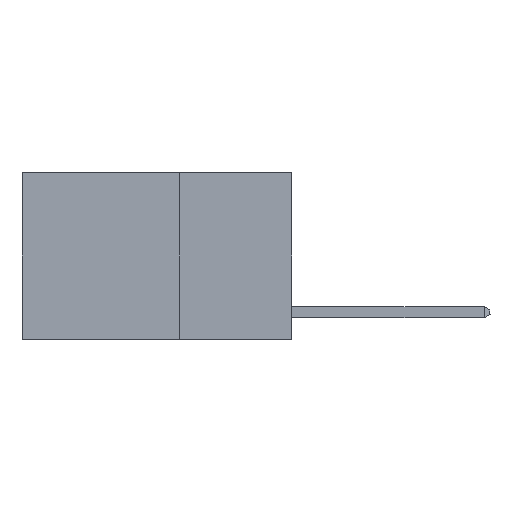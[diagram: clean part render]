
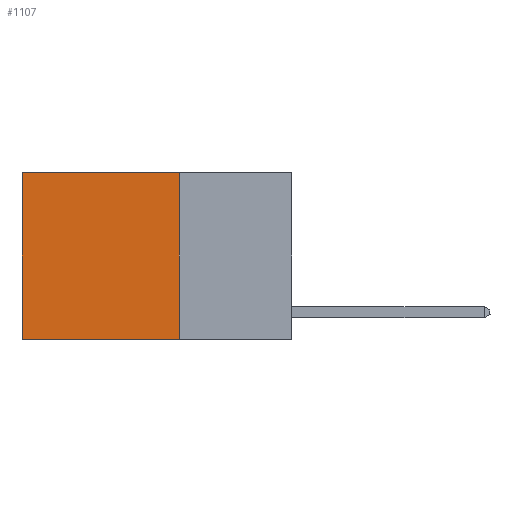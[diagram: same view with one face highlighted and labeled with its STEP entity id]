
A CAD part, left-side view. The second image highlights one B-rep face of the part: STEP entity #1107.
In plain terms, the highlighted planar face has unit normal (-1, 0, 0).
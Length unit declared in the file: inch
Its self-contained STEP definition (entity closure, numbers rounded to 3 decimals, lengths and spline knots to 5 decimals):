
#241 = LINE ( 'NONE', #2129, #24975 ) ;
#943 = FACE_OUTER_BOUND ( 'NONE', #8491, .T. ) ;
#1107 = ADVANCED_FACE ( 'NONE', ( #943 ), #19808, .F. ) ;
#1200 = EDGE_CURVE ( 'NONE', #25346, #14595, #7645, .T. ) ;
#2129 = CARTESIAN_POINT ( 'NONE',  ( 0.2625, 0.25, 0. ) ) ;
#2719 = CARTESIAN_POINT ( 'NONE',  ( 0.2625, 0.25, 0. ) ) ;
#2790 = AXIS2_PLACEMENT_3D ( 'NONE', #7465, #24281, #11390 ) ;
#3312 = ORIENTED_EDGE ( 'NONE', *, *, #1200, .T. ) ;
#3398 = CARTESIAN_POINT ( 'NONE',  ( 0.2625, 0.25, 0. ) ) ;
#6234 = CARTESIAN_POINT ( 'NONE',  ( 0.2625, 0.6, 0. ) ) ;
#7453 = VERTEX_POINT ( 'NONE', #2719 ) ;
#7465 = CARTESIAN_POINT ( 'NONE',  ( 0.2625, 0.25, 0. ) ) ;
#7645 = LINE ( 'NONE', #26067, #15095 ) ;
#7686 = VECTOR ( 'NONE', #24689, 39.37008 ) ;
#8491 = EDGE_LOOP ( 'NONE', ( #3312, #26385, #12675, #25657 ) ) ;
#10450 = DIRECTION ( 'NONE',  ( 0., 0., -1. ) ) ;
#11027 = EDGE_CURVE ( 'NONE', #7453, #25346, #13471, .T. ) ;
#11390 = DIRECTION ( 'NONE',  ( 0., 0., -1. ) ) ;
#12449 = CARTESIAN_POINT ( 'NONE',  ( 0.2625, 0.25, -0.37 ) ) ;
#12675 = ORIENTED_EDGE ( 'NONE', *, *, #24323, .F. ) ;
#13471 = LINE ( 'NONE', #3398, #19526 ) ;
#13715 = DIRECTION ( 'NONE',  ( 0., 0., -1. ) ) ;
#14595 = VERTEX_POINT ( 'NONE', #20973 ) ;
#15095 = VECTOR ( 'NONE', #13715, 39.37008 ) ;
#15436 = VERTEX_POINT ( 'NONE', #12449 ) ;
#16542 = LINE ( 'NONE', #18158, #7686 ) ;
#18158 = CARTESIAN_POINT ( 'NONE',  ( 0.2625, 0.25, -0.37 ) ) ;
#19526 = VECTOR ( 'NONE', #24349, 39.37008 ) ;
#19808 = PLANE ( 'NONE',  #2790 ) ;
#20973 = CARTESIAN_POINT ( 'NONE',  ( 0.2625, 0.6, -0.37 ) ) ;
#24281 = DIRECTION ( 'NONE',  ( 1., 0., 0. ) ) ;
#24323 = EDGE_CURVE ( 'NONE', #7453, #15436, #241, .T. ) ;
#24349 = DIRECTION ( 'NONE',  ( 0., 1., 0. ) ) ;
#24689 = DIRECTION ( 'NONE',  ( 0., 1., 0. ) ) ;
#24975 = VECTOR ( 'NONE', #10450, 39.37008 ) ;
#25346 = VERTEX_POINT ( 'NONE', #6234 ) ;
#25361 = EDGE_CURVE ( 'NONE', #15436, #14595, #16542, .T. ) ;
#25657 = ORIENTED_EDGE ( 'NONE', *, *, #11027, .T. ) ;
#26067 = CARTESIAN_POINT ( 'NONE',  ( 0.2625, 0.6, 0. ) ) ;
#26385 = ORIENTED_EDGE ( 'NONE', *, *, #25361, .F. ) ;
